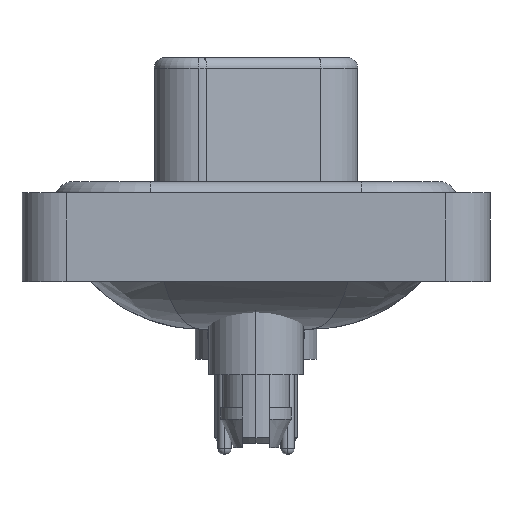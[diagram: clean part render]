
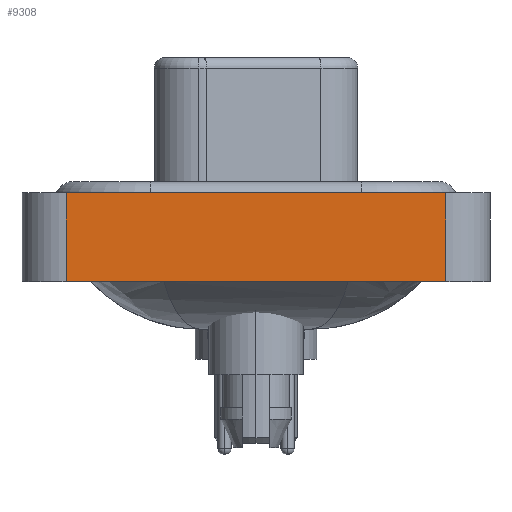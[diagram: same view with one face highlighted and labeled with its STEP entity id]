
A CAD part, left-side view. The second image highlights one B-rep face of the part: STEP entity #9308.
In plain terms, the highlighted planar face has unit normal (-1, 0, 0).
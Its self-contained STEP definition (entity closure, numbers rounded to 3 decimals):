
#559 = DIRECTION ( 'NONE',  ( -1., 0., 0. ) ) ;
#638 = VECTOR ( 'NONE', #5123, 1000. ) ;
#805 = PLANE ( 'NONE',  #16089 ) ;
#966 = LINE ( 'NONE', #8710, #24611 ) ;
#1185 = LINE ( 'NONE', #12602, #638 ) ;
#2239 = EDGE_LOOP ( 'NONE', ( #23933, #6852, #15762, #7624 ) ) ;
#3384 = VERTEX_POINT ( 'NONE', #7017 ) ;
#5123 = DIRECTION ( 'NONE',  ( 0., -1., 0. ) ) ;
#6390 = VERTEX_POINT ( 'NONE', #24235 ) ;
#6852 = ORIENTED_EDGE ( 'NONE', *, *, #14958, .F. ) ;
#7017 = CARTESIAN_POINT ( 'NONE',  ( -7.35, -8.55, 0.4 ) ) ;
#7624 = ORIENTED_EDGE ( 'NONE', *, *, #18252, .T. ) ;
#8710 = CARTESIAN_POINT ( 'NONE',  ( -7.35, 8.55, -3.6 ) ) ;
#8922 = VERTEX_POINT ( 'NONE', #18956 ) ;
#9308 = ADVANCED_FACE ( 'NONE', ( #10198 ), #805, .T. ) ;
#10198 = FACE_OUTER_BOUND ( 'NONE', #2239, .T. ) ;
#11580 = CARTESIAN_POINT ( 'NONE',  ( -7.35, -8.55, -3.6 ) ) ;
#11829 = CARTESIAN_POINT ( 'NONE',  ( -7.35, -8.55, -3.6 ) ) ;
#12317 = LINE ( 'NONE', #11829, #15990 ) ;
#12602 = CARTESIAN_POINT ( 'NONE',  ( -7.35, -8.55, 0.4 ) ) ;
#14958 = EDGE_CURVE ( 'NONE', #6390, #3384, #1185, .T. ) ;
#15250 = CARTESIAN_POINT ( 'NONE',  ( -7.35, -8.55, -3.6 ) ) ;
#15614 = LINE ( 'NONE', #11580, #16159 ) ;
#15762 = ORIENTED_EDGE ( 'NONE', *, *, #19601, .F. ) ;
#15990 = VECTOR ( 'NONE', #23584, 1000. ) ;
#16033 = CARTESIAN_POINT ( 'NONE',  ( -7.35, -8.55, -3.6 ) ) ;
#16089 = AXIS2_PLACEMENT_3D ( 'NONE', #16033, #559, #20789 ) ;
#16159 = VECTOR ( 'NONE', #19163, 1000. ) ;
#16800 = DIRECTION ( 'NONE',  ( 0., 0., 1. ) ) ;
#17993 = VERTEX_POINT ( 'NONE', #15250 ) ;
#18252 = EDGE_CURVE ( 'NONE', #8922, #17993, #12317, .T. ) ;
#18956 = CARTESIAN_POINT ( 'NONE',  ( -7.35, 8.55, -3.6 ) ) ;
#19163 = DIRECTION ( 'NONE',  ( 0., 0., 1. ) ) ;
#19601 = EDGE_CURVE ( 'NONE', #8922, #6390, #966, .T. ) ;
#20757 = EDGE_CURVE ( 'NONE', #17993, #3384, #15614, .T. ) ;
#20789 = DIRECTION ( 'NONE',  ( 0., 0., 1. ) ) ;
#23584 = DIRECTION ( 'NONE',  ( 0., -1., 0. ) ) ;
#23933 = ORIENTED_EDGE ( 'NONE', *, *, #20757, .T. ) ;
#24235 = CARTESIAN_POINT ( 'NONE',  ( -7.35, 8.55, 0.4 ) ) ;
#24611 = VECTOR ( 'NONE', #16800, 1000. ) ;
